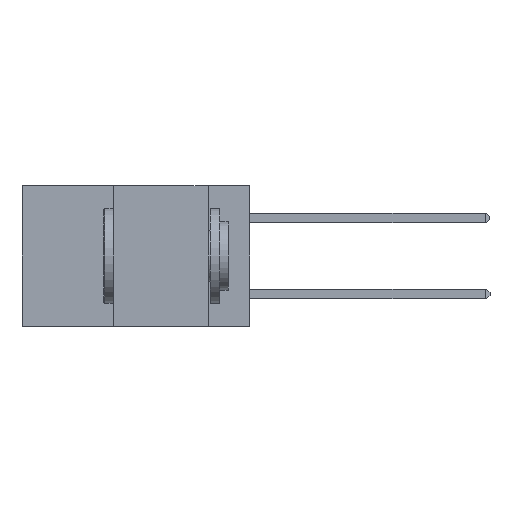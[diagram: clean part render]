
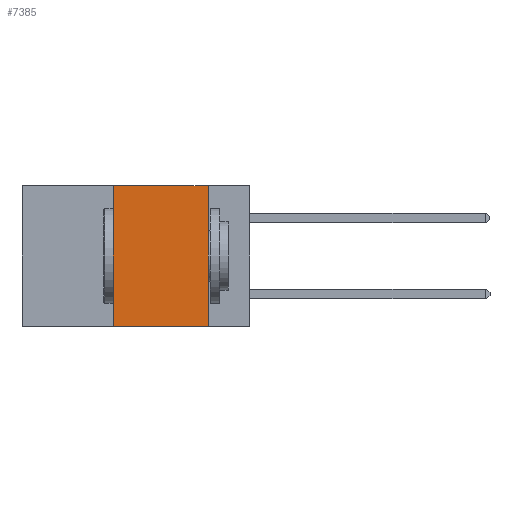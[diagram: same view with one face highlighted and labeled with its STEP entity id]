
A CAD part, left-side view. The second image highlights one B-rep face of the part: STEP entity #7385.
In plain terms, the highlighted planar face has unit normal (-1, 0, 0).
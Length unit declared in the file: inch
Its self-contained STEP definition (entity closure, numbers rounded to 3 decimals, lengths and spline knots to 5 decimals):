
#888 = LINE ( 'NONE', #10009, #14687 ) ;
#1620 = LINE ( 'NONE', #10542, #9966 ) ;
#2246 = VECTOR ( 'NONE', #14630, 39.37008 ) ;
#2356 = DIRECTION ( 'NONE',  ( 1., 0., 0. ) ) ;
#3030 = AXIS2_PLACEMENT_3D ( 'NONE', #12187, #2356, #13857 ) ;
#3451 = CARTESIAN_POINT ( 'NONE',  ( 0., 0.36, -0.37 ) ) ;
#3998 = PLANE ( 'NONE',  #3030 ) ;
#4163 = DIRECTION ( 'NONE',  ( 0., 0., -1. ) ) ;
#4801 = CARTESIAN_POINT ( 'NONE',  ( 0., 0.6, -0.37 ) ) ;
#5159 = FACE_OUTER_BOUND ( 'NONE', #14407, .T. ) ;
#6184 = LINE ( 'NONE', #4801, #2246 ) ;
#7352 = VECTOR ( 'NONE', #4163, 39.37008 ) ;
#7385 = ADVANCED_FACE ( 'NONE', ( #5159 ), #3998, .F. ) ;
#7603 = CARTESIAN_POINT ( 'NONE',  ( 0., 0.11, -0.37 ) ) ;
#9911 = CARTESIAN_POINT ( 'NONE',  ( 0., 0.11, 0. ) ) ;
#9964 = EDGE_CURVE ( 'NONE', #11280, #10416, #6184, .T. ) ;
#9966 = VECTOR ( 'NONE', #12171, 39.37008 ) ;
#10009 = CARTESIAN_POINT ( 'NONE',  ( 0., 0.36, 0. ) ) ;
#10416 = VERTEX_POINT ( 'NONE', #7603 ) ;
#10542 = CARTESIAN_POINT ( 'NONE',  ( 0., 0.6, 0. ) ) ;
#10735 = CARTESIAN_POINT ( 'NONE',  ( 0., 0.11, 0. ) ) ;
#10796 = EDGE_CURVE ( 'NONE', #19402, #21415, #1620, .T. ) ;
#11280 = VERTEX_POINT ( 'NONE', #3451 ) ;
#11299 = CARTESIAN_POINT ( 'NONE',  ( 0., 0.36, 0. ) ) ;
#11647 = LINE ( 'NONE', #10735, #7352 ) ;
#12171 = DIRECTION ( 'NONE',  ( 0., -1., 0. ) ) ;
#12187 = CARTESIAN_POINT ( 'NONE',  ( 0., 0.6, 0. ) ) ;
#13857 = DIRECTION ( 'NONE',  ( 0., 0., -1. ) ) ;
#14407 = EDGE_LOOP ( 'NONE', ( #17704, #17955, #18022, #18476 ) ) ;
#14630 = DIRECTION ( 'NONE',  ( 0., -1., 0. ) ) ;
#14687 = VECTOR ( 'NONE', #16644, 39.37008 ) ;
#16644 = DIRECTION ( 'NONE',  ( 0., 0., 1. ) ) ;
#17704 = ORIENTED_EDGE ( 'NONE', *, *, #18207, .F. ) ;
#17955 = ORIENTED_EDGE ( 'NONE', *, *, #10796, .F. ) ;
#18022 = ORIENTED_EDGE ( 'NONE', *, *, #20235, .F. ) ;
#18207 = EDGE_CURVE ( 'NONE', #21415, #10416, #11647, .T. ) ;
#18476 = ORIENTED_EDGE ( 'NONE', *, *, #9964, .T. ) ;
#19402 = VERTEX_POINT ( 'NONE', #11299 ) ;
#20235 = EDGE_CURVE ( 'NONE', #11280, #19402, #888, .T. ) ;
#21415 = VERTEX_POINT ( 'NONE', #9911 ) ;
